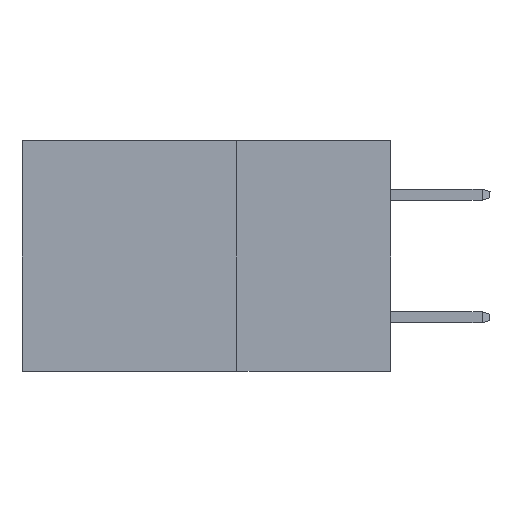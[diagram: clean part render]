
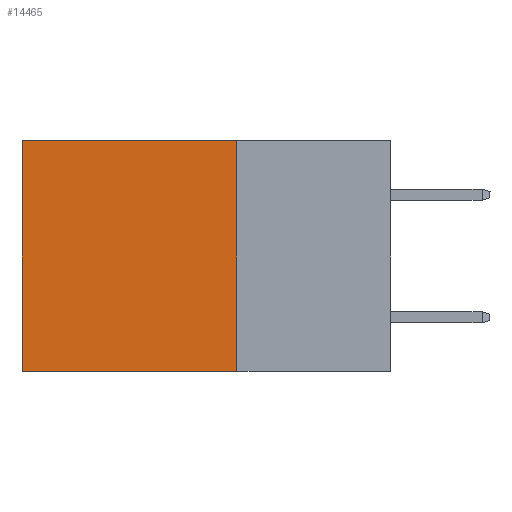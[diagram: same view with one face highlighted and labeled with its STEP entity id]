
A CAD part, left-side view. The second image highlights one B-rep face of the part: STEP entity #14465.
In plain terms, the highlighted planar face has unit normal (-1, 0, 0).
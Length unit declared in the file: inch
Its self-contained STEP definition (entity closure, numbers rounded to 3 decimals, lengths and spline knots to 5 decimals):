
#43 = VECTOR ( 'NONE', #13961, 39.37008 ) ;
#97 = VERTEX_POINT ( 'NONE', #3739 ) ;
#219 = CARTESIAN_POINT ( 'NONE',  ( 0.2875, 0.25, -0.375 ) ) ;
#1271 = ORIENTED_EDGE ( 'NONE', *, *, #8377, .T. ) ;
#1273 = DIRECTION ( 'NONE',  ( 1., 0., 0. ) ) ;
#1309 = LINE ( 'NONE', #7346, #13592 ) ;
#1539 = ORIENTED_EDGE ( 'NONE', *, *, #14666, .F. ) ;
#1559 = ORIENTED_EDGE ( 'NONE', *, *, #13242, .F. ) ;
#1830 = EDGE_LOOP ( 'NONE', ( #14815, #1559, #1539, #1271 ) ) ;
#3244 = CARTESIAN_POINT ( 'NONE',  ( 0.2875, 0.6, 0. ) ) ;
#3484 = CARTESIAN_POINT ( 'NONE',  ( 0.2875, 0.6, -0.375 ) ) ;
#3739 = CARTESIAN_POINT ( 'NONE',  ( 0.2875, 0.25, 0. ) ) ;
#3909 = EDGE_CURVE ( 'NONE', #14337, #13624, #5215, .T. ) ;
#4488 = CARTESIAN_POINT ( 'NONE',  ( 0.2875, 0.25, -0.375 ) ) ;
#4817 = DIRECTION ( 'NONE',  ( 0., 0., -1. ) ) ;
#5215 = LINE ( 'NONE', #8701, #7655 ) ;
#5621 = AXIS2_PLACEMENT_3D ( 'NONE', #5657, #1273, #5884 ) ;
#5657 = CARTESIAN_POINT ( 'NONE',  ( 0.2875, 0.25, -0.375 ) ) ;
#5884 = DIRECTION ( 'NONE',  ( 0., 0., -1. ) ) ;
#6062 = DIRECTION ( 'NONE',  ( 0., 1., 0. ) ) ;
#6785 = FACE_OUTER_BOUND ( 'NONE', #1830, .T. ) ;
#7346 = CARTESIAN_POINT ( 'NONE',  ( 0.2875, 0.25, 0. ) ) ;
#7655 = VECTOR ( 'NONE', #13320, 39.37008 ) ;
#8301 = VECTOR ( 'NONE', #4817, 39.37008 ) ;
#8377 = EDGE_CURVE ( 'NONE', #97, #14337, #1309, .T. ) ;
#8701 = CARTESIAN_POINT ( 'NONE',  ( 0.2875, 0.6, -0.375 ) ) ;
#9596 = LINE ( 'NONE', #219, #8301 ) ;
#10243 = LINE ( 'NONE', #4488, #43 ) ;
#11560 = PLANE ( 'NONE',  #5621 ) ;
#13242 = EDGE_CURVE ( 'NONE', #14334, #13624, #10243, .T. ) ;
#13320 = DIRECTION ( 'NONE',  ( 0., 0., -1. ) ) ;
#13592 = VECTOR ( 'NONE', #6062, 39.37008 ) ;
#13624 = VERTEX_POINT ( 'NONE', #3484 ) ;
#13961 = DIRECTION ( 'NONE',  ( 0., 1., 0. ) ) ;
#14334 = VERTEX_POINT ( 'NONE', #14687 ) ;
#14337 = VERTEX_POINT ( 'NONE', #3244 ) ;
#14465 = ADVANCED_FACE ( 'NONE', ( #6785 ), #11560, .F. ) ;
#14666 = EDGE_CURVE ( 'NONE', #97, #14334, #9596, .T. ) ;
#14687 = CARTESIAN_POINT ( 'NONE',  ( 0.2875, 0.25, -0.375 ) ) ;
#14815 = ORIENTED_EDGE ( 'NONE', *, *, #3909, .T. ) ;
